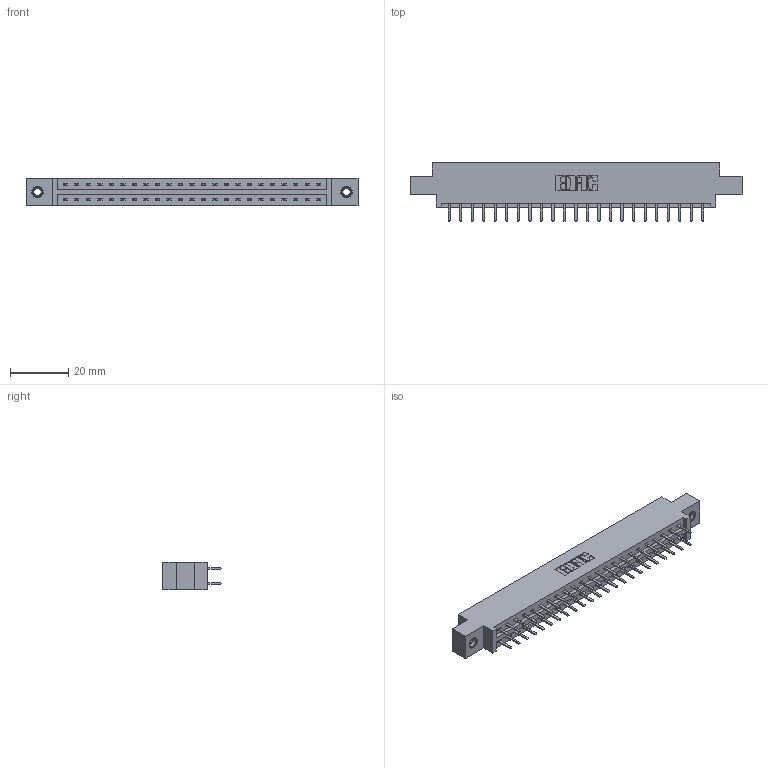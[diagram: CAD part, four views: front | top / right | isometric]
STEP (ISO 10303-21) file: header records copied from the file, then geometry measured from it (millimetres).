
FILE_DESCRIPTION (( 'STEP AP203' ), '1' );
FILE_NAME ('387-046-520-807.STEP', '2019-10-18T06:57:44', ( '' ), ( '' ), 'SwSTEP 2.0', 'SolidWorks 2016', '' );
FILE_SCHEMA (( 'CONFIG_CONTROL_DESIGN' ));
Length unit declared in the file: inch
Products named in the file (4): 337 Part_0.170 Offset - 0.156 Dia-TI; 345-292-001_345-293-120; 345-250-001_345-250-005-103; 387-046-520-807
Assembly tree (49 placements, depth 2):
  387-046-520-807
    337 Part_0.170 Offset - 0.156 Dia-TI
    345-292-001_345-293-120  x46
    345-250-001_345-250-005-103  x2
Bounding box: 114.15 x 20.02 x 9.4 mm (x, y, z)
Volume: 11625.6 mm3; surface area: 13044.3 mm2
Topology: 49 solids, 49 shells, 2846 faces, 8233 edges, 5358 vertices
Faces by surface type: plane 1946, cylinder 884, cone 12, torus 4
Entity records: 21722 total; most frequent: CARTESIAN_POINT 3669, ORIENTED_EDGE 3586, DIRECTION 3175, EDGE_CURVE 1793, VECTOR 1641, LINE 1641, VERTEX_POINT 1188, AXIS2_PLACEMENT_3D 767
